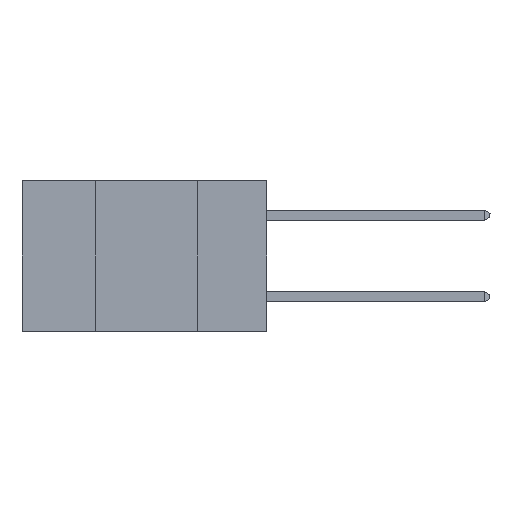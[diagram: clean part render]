
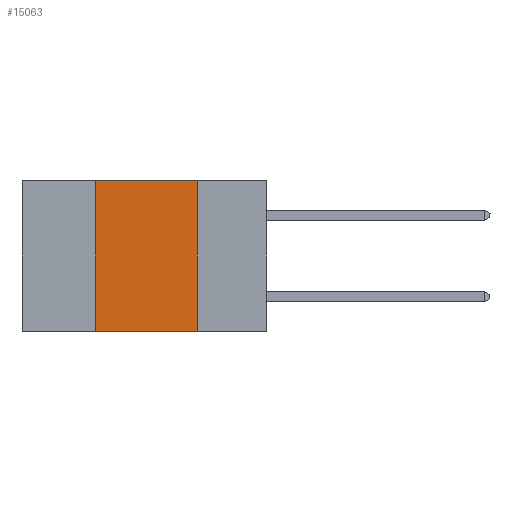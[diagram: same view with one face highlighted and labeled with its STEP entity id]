
A CAD part, left-side view. The second image highlights one B-rep face of the part: STEP entity #15063.
In plain terms, the highlighted planar face has unit normal (-1, 0, 0).
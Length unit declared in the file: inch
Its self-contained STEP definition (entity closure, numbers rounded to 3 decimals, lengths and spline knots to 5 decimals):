
#2794 = CARTESIAN_POINT ( 'NONE',  ( 0., 0.17, 0. ) ) ;
#2808 = EDGE_CURVE ( 'NONE', #22330, #4416, #6483, .T. ) ;
#4416 = VERTEX_POINT ( 'NONE', #10174 ) ;
#4771 = VERTEX_POINT ( 'NONE', #31947 ) ;
#5665 = CARTESIAN_POINT ( 'NONE',  ( 0., 0.6, 0. ) ) ;
#5852 = VECTOR ( 'NONE', #30502, 39.37008 ) ;
#6483 = LINE ( 'NONE', #14321, #16890 ) ;
#6993 = DIRECTION ( 'NONE',  ( 1., 0., 0. ) ) ;
#8420 = DIRECTION ( 'NONE',  ( 0., 0., 1. ) ) ;
#8585 = EDGE_LOOP ( 'NONE', ( #32017, #26067, #25550, #13700 ) ) ;
#10174 = CARTESIAN_POINT ( 'NONE',  ( 0., 0.17, -0.37 ) ) ;
#11079 = LINE ( 'NONE', #25896, #17011 ) ;
#13051 = CARTESIAN_POINT ( 'NONE',  ( 0., 0.17, 0. ) ) ;
#13326 = CARTESIAN_POINT ( 'NONE',  ( 0., 0.42, -0.37 ) ) ;
#13700 = ORIENTED_EDGE ( 'NONE', *, *, #2808, .T. ) ;
#14321 = CARTESIAN_POINT ( 'NONE',  ( 0., 0.6, -0.37 ) ) ;
#15063 = ADVANCED_FACE ( 'NONE', ( #17149 ), #21965, .F. ) ;
#16890 = VECTOR ( 'NONE', #24791, 39.37008 ) ;
#17011 = VECTOR ( 'NONE', #8420, 39.37008 ) ;
#17149 = FACE_OUTER_BOUND ( 'NONE', #8585, .T. ) ;
#17306 = CARTESIAN_POINT ( 'NONE',  ( 0., 0.6, 0. ) ) ;
#17558 = LINE ( 'NONE', #13051, #26948 ) ;
#17823 = EDGE_CURVE ( 'NONE', #21353, #4416, #17558, .T. ) ;
#20373 = DIRECTION ( 'NONE',  ( 0., 0., -1. ) ) ;
#21353 = VERTEX_POINT ( 'NONE', #2794 ) ;
#21965 = PLANE ( 'NONE',  #32240 ) ;
#22330 = VERTEX_POINT ( 'NONE', #13326 ) ;
#24791 = DIRECTION ( 'NONE',  ( 0., -1., 0. ) ) ;
#25550 = ORIENTED_EDGE ( 'NONE', *, *, #26631, .F. ) ;
#25896 = CARTESIAN_POINT ( 'NONE',  ( 0., 0.42, 0. ) ) ;
#26067 = ORIENTED_EDGE ( 'NONE', *, *, #27609, .F. ) ;
#26631 = EDGE_CURVE ( 'NONE', #22330, #4771, #11079, .T. ) ;
#26948 = VECTOR ( 'NONE', #20373, 39.37008 ) ;
#27289 = DIRECTION ( 'NONE',  ( 0., 0., -1. ) ) ;
#27609 = EDGE_CURVE ( 'NONE', #4771, #21353, #30986, .T. ) ;
#30502 = DIRECTION ( 'NONE',  ( 0., -1., 0. ) ) ;
#30986 = LINE ( 'NONE', #5665, #5852 ) ;
#31947 = CARTESIAN_POINT ( 'NONE',  ( 0., 0.42, 0. ) ) ;
#32017 = ORIENTED_EDGE ( 'NONE', *, *, #17823, .F. ) ;
#32240 = AXIS2_PLACEMENT_3D ( 'NONE', #17306, #6993, #27289 ) ;
